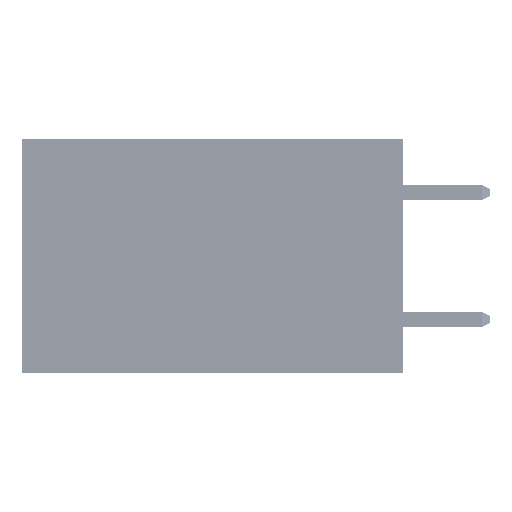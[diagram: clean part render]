
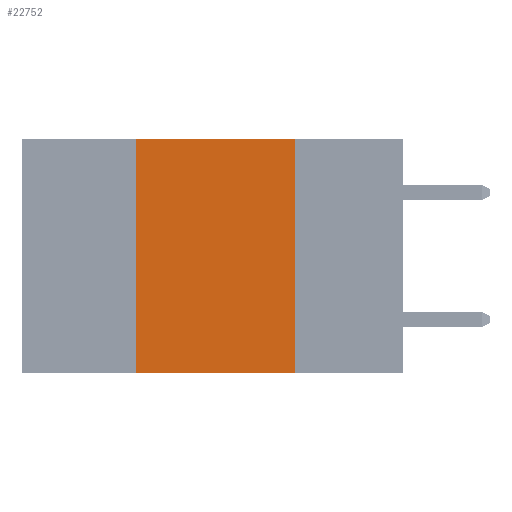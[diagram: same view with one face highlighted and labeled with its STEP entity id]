
A CAD part, left-side view. The second image highlights one B-rep face of the part: STEP entity #22752.
In plain terms, the highlighted planar face has unit normal (-1, 0, 0).
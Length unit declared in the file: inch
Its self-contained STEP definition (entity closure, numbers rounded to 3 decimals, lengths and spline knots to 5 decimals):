
#528 = EDGE_CURVE ( 'NONE', #6594, #33884, #42894, .T. ) ;
#2218 = VECTOR ( 'NONE', #31922, 39.37008 ) ;
#2241 = CARTESIAN_POINT ( 'NONE',  ( 0., 0.6, 0. ) ) ;
#6331 = ORIENTED_EDGE ( 'NONE', *, *, #528, .F. ) ;
#6594 = VERTEX_POINT ( 'NONE', #43204 ) ;
#6618 = EDGE_CURVE ( 'NONE', #25515, #6594, #25012, .T. ) ;
#8334 = CARTESIAN_POINT ( 'NONE',  ( 0., 0.42, 0. ) ) ;
#8999 = ORIENTED_EDGE ( 'NONE', *, *, #6618, .F. ) ;
#10203 = DIRECTION ( 'NONE',  ( 0., 0., -1. ) ) ;
#13055 = CARTESIAN_POINT ( 'NONE',  ( 0., 0.6, -0.37 ) ) ;
#15144 = CARTESIAN_POINT ( 'NONE',  ( 0., 0.42, -0.37 ) ) ;
#15212 = DIRECTION ( 'NONE',  ( 0., 0., -1. ) ) ;
#15868 = EDGE_LOOP ( 'NONE', ( #6331, #8999, #32489, #37882 ) ) ;
#16332 = LINE ( 'NONE', #46516, #2218 ) ;
#20597 = DIRECTION ( 'NONE',  ( 0., -1., 0. ) ) ;
#20885 = VECTOR ( 'NONE', #24483, 39.37008 ) ;
#22752 = ADVANCED_FACE ( 'NONE', ( #37699 ), #24683, .F. ) ;
#24483 = DIRECTION ( 'NONE',  ( 0., -1., 0. ) ) ;
#24683 = PLANE ( 'NONE',  #32931 ) ;
#25012 = LINE ( 'NONE', #2241, #20885 ) ;
#25515 = VERTEX_POINT ( 'NONE', #8334 ) ;
#26268 = CARTESIAN_POINT ( 'NONE',  ( 0., 0.17, 0. ) ) ;
#27390 = LINE ( 'NONE', #13055, #31486 ) ;
#28075 = VERTEX_POINT ( 'NONE', #15144 ) ;
#28847 = VECTOR ( 'NONE', #15212, 39.37008 ) ;
#31486 = VECTOR ( 'NONE', #20597, 39.37008 ) ;
#31922 = DIRECTION ( 'NONE',  ( 0., 0., 1. ) ) ;
#32268 = CARTESIAN_POINT ( 'NONE',  ( 0., 0.6, 0. ) ) ;
#32489 = ORIENTED_EDGE ( 'NONE', *, *, #38240, .F. ) ;
#32931 = AXIS2_PLACEMENT_3D ( 'NONE', #32268, #47681, #10203 ) ;
#33884 = VERTEX_POINT ( 'NONE', #47353 ) ;
#37699 = FACE_OUTER_BOUND ( 'NONE', #15868, .T. ) ;
#37882 = ORIENTED_EDGE ( 'NONE', *, *, #47306, .T. ) ;
#38240 = EDGE_CURVE ( 'NONE', #28075, #25515, #16332, .T. ) ;
#42894 = LINE ( 'NONE', #26268, #28847 ) ;
#43204 = CARTESIAN_POINT ( 'NONE',  ( 0., 0.17, 0. ) ) ;
#46516 = CARTESIAN_POINT ( 'NONE',  ( 0., 0.42, 0. ) ) ;
#47306 = EDGE_CURVE ( 'NONE', #28075, #33884, #27390, .T. ) ;
#47353 = CARTESIAN_POINT ( 'NONE',  ( 0., 0.17, -0.37 ) ) ;
#47681 = DIRECTION ( 'NONE',  ( 1., 0., 0. ) ) ;
